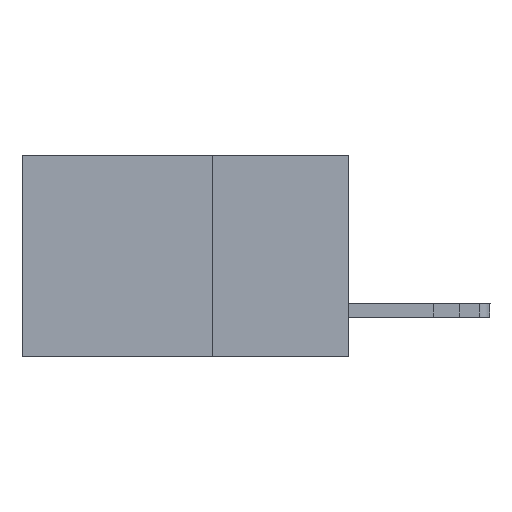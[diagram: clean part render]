
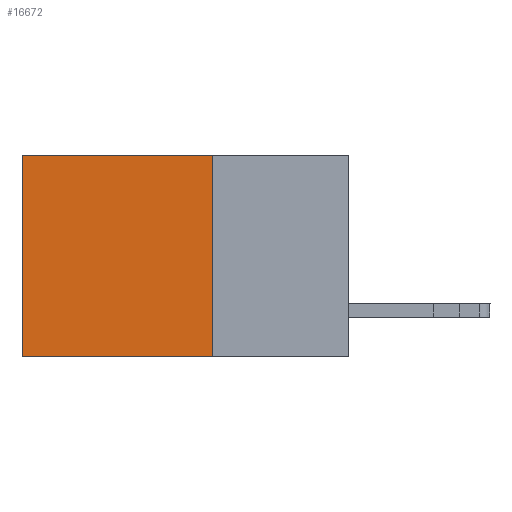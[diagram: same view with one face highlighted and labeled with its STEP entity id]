
A CAD part, left-side view. The second image highlights one B-rep face of the part: STEP entity #16672.
In plain terms, the highlighted planar face has unit normal (-1, 0, 0).
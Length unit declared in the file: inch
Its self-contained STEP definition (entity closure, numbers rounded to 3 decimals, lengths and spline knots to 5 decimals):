
#1317 = VERTEX_POINT ( 'NONE', #2858 ) ;
#1354 = VECTOR ( 'NONE', #17372, 39.37008 ) ;
#1773 = LINE ( 'NONE', #7742, #1354 ) ;
#1849 = DIRECTION ( 'NONE',  ( 0., 0., -1. ) ) ;
#2242 = VECTOR ( 'NONE', #1849, 39.37008 ) ;
#2331 = EDGE_LOOP ( 'NONE', ( #14943, #6565, #10920, #7976 ) ) ;
#2840 = EDGE_CURVE ( 'NONE', #8327, #10932, #4990, .T. ) ;
#2858 = CARTESIAN_POINT ( 'NONE',  ( 0.298, 0.6, -0.37 ) ) ;
#2940 = PLANE ( 'NONE',  #16504 ) ;
#3088 = CARTESIAN_POINT ( 'NONE',  ( 0.298, 0.25, 0. ) ) ;
#3663 = VECTOR ( 'NONE', #4316, 39.37008 ) ;
#4316 = DIRECTION ( 'NONE',  ( 0., 1., 0. ) ) ;
#4636 = CARTESIAN_POINT ( 'NONE',  ( 0.298, 0.6, 0. ) ) ;
#4885 = CARTESIAN_POINT ( 'NONE',  ( 0.298, 0.25, 0. ) ) ;
#4990 = LINE ( 'NONE', #3088, #2242 ) ;
#6565 = ORIENTED_EDGE ( 'NONE', *, *, #17572, .F. ) ;
#6712 = CARTESIAN_POINT ( 'NONE',  ( 0.298, 0.25, -0.37 ) ) ;
#7330 = CARTESIAN_POINT ( 'NONE',  ( 0.298, 0.25, 0. ) ) ;
#7742 = CARTESIAN_POINT ( 'NONE',  ( 0.298, 0.6, 0. ) ) ;
#7976 = ORIENTED_EDGE ( 'NONE', *, *, #17166, .T. ) ;
#8327 = VERTEX_POINT ( 'NONE', #4885 ) ;
#10571 = CARTESIAN_POINT ( 'NONE',  ( 0.298, 0.25, -0.37 ) ) ;
#10920 = ORIENTED_EDGE ( 'NONE', *, *, #2840, .F. ) ;
#10932 = VERTEX_POINT ( 'NONE', #10571 ) ;
#11149 = CARTESIAN_POINT ( 'NONE',  ( 0.298, 0.25, 0. ) ) ;
#11153 = FACE_OUTER_BOUND ( 'NONE', #2331, .T. ) ;
#11788 = VECTOR ( 'NONE', #16817, 39.37008 ) ;
#12216 = LINE ( 'NONE', #7330, #11788 ) ;
#12298 = VERTEX_POINT ( 'NONE', #4636 ) ;
#12537 = DIRECTION ( 'NONE',  ( 1., 0., 0. ) ) ;
#13963 = DIRECTION ( 'NONE',  ( 0., 0., -1. ) ) ;
#14943 = ORIENTED_EDGE ( 'NONE', *, *, #16846, .T. ) ;
#16504 = AXIS2_PLACEMENT_3D ( 'NONE', #11149, #12537, #13963 ) ;
#16672 = ADVANCED_FACE ( 'NONE', ( #11153 ), #2940, .F. ) ;
#16817 = DIRECTION ( 'NONE',  ( 0., 1., 0. ) ) ;
#16846 = EDGE_CURVE ( 'NONE', #12298, #1317, #1773, .T. ) ;
#17166 = EDGE_CURVE ( 'NONE', #8327, #12298, #12216, .T. ) ;
#17372 = DIRECTION ( 'NONE',  ( 0., 0., -1. ) ) ;
#17500 = LINE ( 'NONE', #6712, #3663 ) ;
#17572 = EDGE_CURVE ( 'NONE', #10932, #1317, #17500, .T. ) ;
